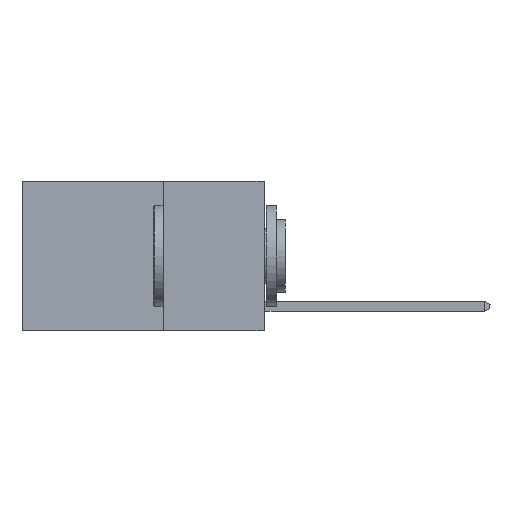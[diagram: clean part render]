
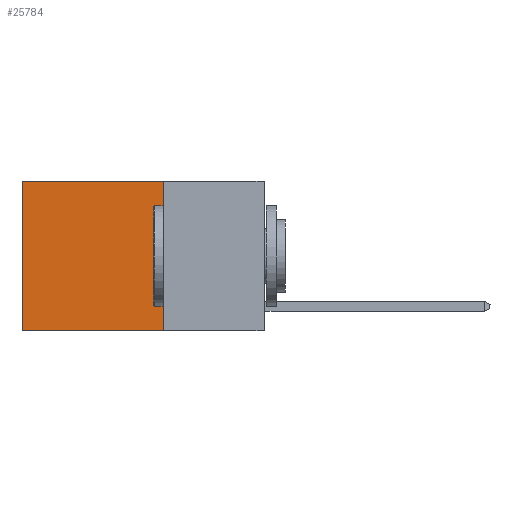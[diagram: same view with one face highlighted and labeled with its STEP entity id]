
A CAD part, left-side view. The second image highlights one B-rep face of the part: STEP entity #25784.
In plain terms, the highlighted planar face has unit normal (-1, 0, 0).
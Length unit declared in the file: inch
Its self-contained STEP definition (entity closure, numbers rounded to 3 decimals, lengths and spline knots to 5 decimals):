
#764 = DIRECTION ( 'NONE',  ( 1., 0., 0. ) ) ;
#1948 = AXIS2_PLACEMENT_3D ( 'NONE', #4832, #764, #23395 ) ;
#1989 = VECTOR ( 'NONE', #2516, 39.37008 ) ;
#2516 = DIRECTION ( 'NONE',  ( 0., 1., 0. ) ) ;
#3151 = DIRECTION ( 'NONE',  ( 0., 1., 0. ) ) ;
#4072 = EDGE_LOOP ( 'NONE', ( #19223, #11984, #6542, #24798 ) ) ;
#4257 = FACE_OUTER_BOUND ( 'NONE', #4072, .T. ) ;
#4832 = CARTESIAN_POINT ( 'NONE',  ( 0.2625, 0.25, 0. ) ) ;
#5161 = CARTESIAN_POINT ( 'NONE',  ( 0.2625, 0.25, 0. ) ) ;
#6536 = LINE ( 'NONE', #21018, #1989 ) ;
#6542 = ORIENTED_EDGE ( 'NONE', *, *, #23236, .F. ) ;
#7940 = DIRECTION ( 'NONE',  ( 0., 0., -1. ) ) ;
#8317 = CARTESIAN_POINT ( 'NONE',  ( 0.2625, 0.25, 0. ) ) ;
#8785 = LINE ( 'NONE', #24426, #20386 ) ;
#8821 = DIRECTION ( 'NONE',  ( 0., 0., -1. ) ) ;
#9229 = CARTESIAN_POINT ( 'NONE',  ( 0.2625, 0.6, -0.37 ) ) ;
#9370 = VERTEX_POINT ( 'NONE', #18417 ) ;
#10086 = EDGE_CURVE ( 'NONE', #22022, #14395, #6536, .T. ) ;
#10349 = EDGE_CURVE ( 'NONE', #9370, #19816, #26513, .T. ) ;
#11984 = ORIENTED_EDGE ( 'NONE', *, *, #10349, .F. ) ;
#14298 = EDGE_CURVE ( 'NONE', #14395, #19816, #8785, .T. ) ;
#14395 = VERTEX_POINT ( 'NONE', #14833 ) ;
#14833 = CARTESIAN_POINT ( 'NONE',  ( 0.2625, 0.6, 0. ) ) ;
#15600 = VECTOR ( 'NONE', #8821, 39.37008 ) ;
#17774 = CARTESIAN_POINT ( 'NONE',  ( 0.2625, 0.25, -0.37 ) ) ;
#18417 = CARTESIAN_POINT ( 'NONE',  ( 0.2625, 0.25, -0.37 ) ) ;
#19223 = ORIENTED_EDGE ( 'NONE', *, *, #14298, .T. ) ;
#19816 = VERTEX_POINT ( 'NONE', #9229 ) ;
#20386 = VECTOR ( 'NONE', #7940, 39.37008 ) ;
#21018 = CARTESIAN_POINT ( 'NONE',  ( 0.2625, 0.25, 0. ) ) ;
#21064 = LINE ( 'NONE', #8317, #15600 ) ;
#22022 = VERTEX_POINT ( 'NONE', #5161 ) ;
#22307 = VECTOR ( 'NONE', #3151, 39.37008 ) ;
#23236 = EDGE_CURVE ( 'NONE', #22022, #9370, #21064, .T. ) ;
#23395 = DIRECTION ( 'NONE',  ( 0., 0., -1. ) ) ;
#23485 = PLANE ( 'NONE',  #1948 ) ;
#24426 = CARTESIAN_POINT ( 'NONE',  ( 0.2625, 0.6, 0. ) ) ;
#24798 = ORIENTED_EDGE ( 'NONE', *, *, #10086, .T. ) ;
#25784 = ADVANCED_FACE ( 'NONE', ( #4257 ), #23485, .F. ) ;
#26513 = LINE ( 'NONE', #17774, #22307 ) ;
